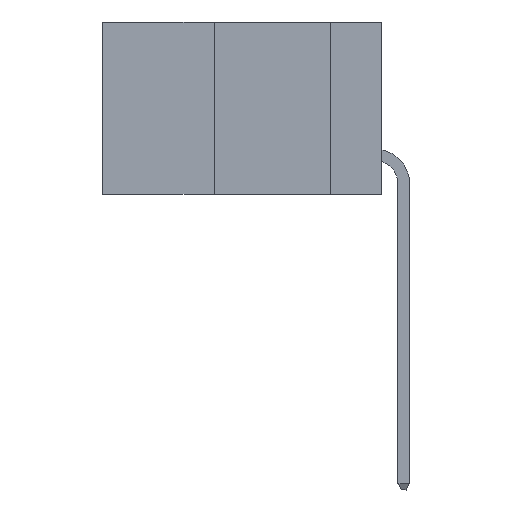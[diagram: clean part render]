
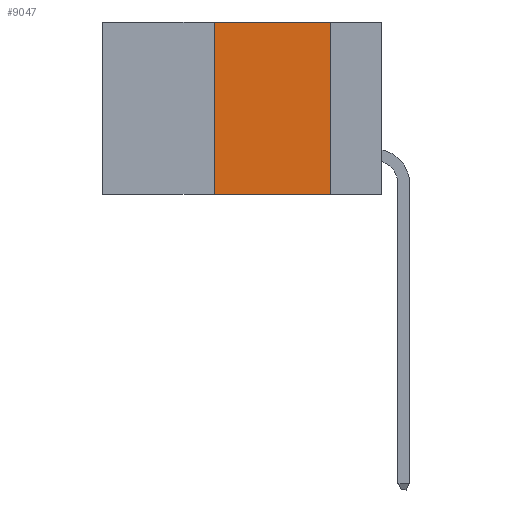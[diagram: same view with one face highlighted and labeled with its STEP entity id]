
A CAD part, left-side view. The second image highlights one B-rep face of the part: STEP entity #9047.
In plain terms, the highlighted planar face has unit normal (-1, 0, 0).
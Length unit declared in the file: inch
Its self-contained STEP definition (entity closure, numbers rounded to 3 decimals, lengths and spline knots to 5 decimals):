
#290 = VERTEX_POINT ( 'NONE', #1705 ) ;
#671 = VECTOR ( 'NONE', #8934, 39.37008 ) ;
#1002 = LINE ( 'NONE', #5512, #7949 ) ;
#1418 = ORIENTED_EDGE ( 'NONE', *, *, #2769, .F. ) ;
#1616 = VECTOR ( 'NONE', #6521, 39.37008 ) ;
#1705 = CARTESIAN_POINT ( 'NONE',  ( 0., 0.36, 0. ) ) ;
#2176 = VECTOR ( 'NONE', #7239, 39.37008 ) ;
#2182 = LINE ( 'NONE', #2318, #1616 ) ;
#2318 = CARTESIAN_POINT ( 'NONE',  ( 0., 0.11, 0. ) ) ;
#2732 = CARTESIAN_POINT ( 'NONE',  ( 0., 0.36, -0.37 ) ) ;
#2747 = ORIENTED_EDGE ( 'NONE', *, *, #8279, .F. ) ;
#2769 = EDGE_CURVE ( 'NONE', #5355, #3124, #2182, .T. ) ;
#2787 = CARTESIAN_POINT ( 'NONE',  ( 0., 0.11, -0.37 ) ) ;
#2819 = CARTESIAN_POINT ( 'NONE',  ( 0., 0.11, 0. ) ) ;
#3124 = VERTEX_POINT ( 'NONE', #2787 ) ;
#3141 = LINE ( 'NONE', #6040, #671 ) ;
#3179 = ORIENTED_EDGE ( 'NONE', *, *, #7337, .T. ) ;
#3464 = CARTESIAN_POINT ( 'NONE',  ( 0., 0.6, 0. ) ) ;
#4162 = AXIS2_PLACEMENT_3D ( 'NONE', #3464, #4982, #5694 ) ;
#4982 = DIRECTION ( 'NONE',  ( 1., 0., 0. ) ) ;
#5329 = DIRECTION ( 'NONE',  ( 0., 0., 1. ) ) ;
#5355 = VERTEX_POINT ( 'NONE', #2819 ) ;
#5512 = CARTESIAN_POINT ( 'NONE',  ( 0., 0.36, 0. ) ) ;
#5694 = DIRECTION ( 'NONE',  ( 0., 0., -1. ) ) ;
#5718 = CARTESIAN_POINT ( 'NONE',  ( 0., 0.6, 0. ) ) ;
#6040 = CARTESIAN_POINT ( 'NONE',  ( 0., 0.6, -0.37 ) ) ;
#6521 = DIRECTION ( 'NONE',  ( 0., 0., -1. ) ) ;
#6595 = VERTEX_POINT ( 'NONE', #2732 ) ;
#6860 = ORIENTED_EDGE ( 'NONE', *, *, #8463, .F. ) ;
#7123 = FACE_OUTER_BOUND ( 'NONE', #8553, .T. ) ;
#7239 = DIRECTION ( 'NONE',  ( 0., -1., 0. ) ) ;
#7337 = EDGE_CURVE ( 'NONE', #6595, #3124, #3141, .T. ) ;
#7762 = LINE ( 'NONE', #5718, #2176 ) ;
#7949 = VECTOR ( 'NONE', #5329, 39.37008 ) ;
#8279 = EDGE_CURVE ( 'NONE', #290, #5355, #7762, .T. ) ;
#8463 = EDGE_CURVE ( 'NONE', #6595, #290, #1002, .T. ) ;
#8553 = EDGE_LOOP ( 'NONE', ( #1418, #2747, #6860, #3179 ) ) ;
#8934 = DIRECTION ( 'NONE',  ( 0., -1., 0. ) ) ;
#9047 = ADVANCED_FACE ( 'NONE', ( #7123 ), #9208, .F. ) ;
#9208 = PLANE ( 'NONE',  #4162 ) ;
